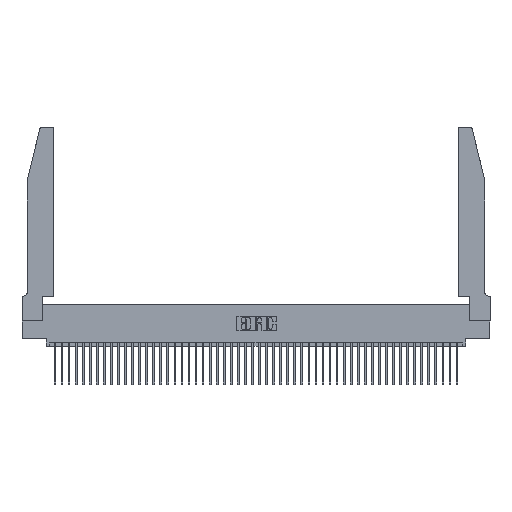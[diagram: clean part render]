
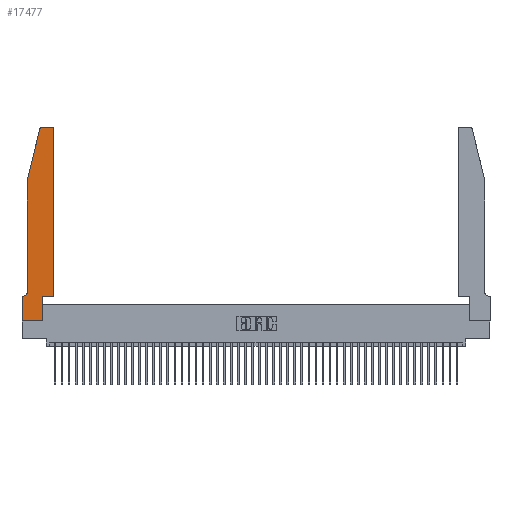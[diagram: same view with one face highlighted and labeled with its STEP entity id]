
A CAD part, top view. The second image highlights one B-rep face of the part: STEP entity #17477.
In plain terms, the highlighted planar face has unit normal (0, 0, 1).
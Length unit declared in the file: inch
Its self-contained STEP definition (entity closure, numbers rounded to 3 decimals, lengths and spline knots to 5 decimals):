
#53 = VERTEX_POINT ( 'NONE', #31183 ) ;
#1269 = CIRCLE ( 'NONE', #37460, 0.03 ) ;
#1338 = CARTESIAN_POINT ( 'NONE',  ( 0.4505, 0.35, 0.37 ) ) ;
#1360 = DIRECTION ( 'NONE',  ( 0., 0., 1. ) ) ;
#1592 = VECTOR ( 'NONE', #30596, 39.37008 ) ;
#1834 = VERTEX_POINT ( 'NONE', #38610 ) ;
#2089 = ORIENTED_EDGE ( 'NONE', *, *, #30046, .T. ) ;
#3142 = VERTEX_POINT ( 'NONE', #16847 ) ;
#4029 = EDGE_CURVE ( 'NONE', #45872, #11763, #17822, .T. ) ;
#4580 = ORIENTED_EDGE ( 'NONE', *, *, #7822, .T. ) ;
#5085 = PLANE ( 'NONE',  #37215 ) ;
#5420 = EDGE_CURVE ( 'NONE', #19648, #16205, #38707, .T. ) ;
#5637 = VERTEX_POINT ( 'NONE', #30866 ) ;
#6032 = ORIENTED_EDGE ( 'NONE', *, *, #9380, .T. ) ;
#7026 = ORIENTED_EDGE ( 'NONE', *, *, #36042, .T. ) ;
#7822 = EDGE_CURVE ( 'NONE', #3142, #5637, #47270, .T. ) ;
#8470 = VECTOR ( 'NONE', #11796, 39.37008 ) ;
#8749 = CARTESIAN_POINT ( 'NONE',  ( 0.2865, 0.35, 0.37 ) ) ;
#9177 = CARTESIAN_POINT ( 'NONE',  ( 0.0055, 0.42, 0.37 ) ) ;
#9285 = EDGE_CURVE ( 'NONE', #36598, #53, #1269, .T. ) ;
#9380 = EDGE_CURVE ( 'NONE', #31233, #19648, #23908, .T. ) ;
#9903 = ORIENTED_EDGE ( 'NONE', *, *, #30215, .T. ) ;
#10704 = VERTEX_POINT ( 'NONE', #27203 ) ;
#11409 = LINE ( 'NONE', #30130, #20197 ) ;
#11763 = VERTEX_POINT ( 'NONE', #32856 ) ;
#11796 = DIRECTION ( 'NONE',  ( -1., 0., 0. ) ) ;
#12970 = EDGE_CURVE ( 'NONE', #10704, #45872, #26565, .T. ) ;
#13613 = VERTEX_POINT ( 'NONE', #40194 ) ;
#15074 = VECTOR ( 'NONE', #30107, 39.37008 ) ;
#15516 = CARTESIAN_POINT ( 'NONE',  ( 0.4505, 0.35, 0.37 ) ) ;
#15694 = DIRECTION ( 'NONE',  ( 1., 0., 0. ) ) ;
#16205 = VERTEX_POINT ( 'NONE', #39256 ) ;
#16847 = CARTESIAN_POINT ( 'NONE',  ( 0.2865, 0., 0.37 ) ) ;
#17477 = ADVANCED_FACE ( 'NONE', ( #25300 ), #5085, .T. ) ;
#17822 = CIRCLE ( 'NONE', #23150, 0.03 ) ;
#17954 = ORIENTED_EDGE ( 'NONE', *, *, #9285, .T. ) ;
#19648 = VERTEX_POINT ( 'NONE', #41262 ) ;
#20080 = DIRECTION ( 'NONE',  ( 1., 0., 0. ) ) ;
#20197 = VECTOR ( 'NONE', #45493, 39.37008 ) ;
#20607 = VECTOR ( 'NONE', #45536, 39.37008 ) ;
#20691 = VECTOR ( 'NONE', #45403, 39.37008 ) ;
#21828 = LINE ( 'NONE', #23031, #20691 ) ;
#23022 = EDGE_CURVE ( 'NONE', #16205, #13613, #11409, .T. ) ;
#23031 = CARTESIAN_POINT ( 'NONE',  ( 0.0755, 2., 0.37 ) ) ;
#23150 = AXIS2_PLACEMENT_3D ( 'NONE', #26439, #41498, #15694 ) ;
#23663 = DIRECTION ( 'NONE',  ( 0., 0., -1. ) ) ;
#23764 = CARTESIAN_POINT ( 'NONE',  ( 0., 0.35, 0.37 ) ) ;
#23908 = CIRCLE ( 'NONE', #37174, 0.07 ) ;
#24202 = EDGE_CURVE ( 'NONE', #53, #1834, #21828, .T. ) ;
#24320 = ORIENTED_EDGE ( 'NONE', *, *, #23022, .T. ) ;
#24430 = CARTESIAN_POINT ( 'NONE',  ( 0.284, 2.72, 0.37 ) ) ;
#25300 = FACE_OUTER_BOUND ( 'NONE', #26370, .T. ) ;
#26370 = EDGE_LOOP ( 'NONE', ( #7026, #17954, #39150, #9903, #6032, #30390, #24320, #47570, #4580, #2089, #48081, #40801 ) ) ;
#26439 = CARTESIAN_POINT ( 'NONE',  ( 0.4205, 2.72, 0.37 ) ) ;
#26565 = LINE ( 'NONE', #1338, #48169 ) ;
#26760 = CARTESIAN_POINT ( 'NONE',  ( 0.4505, 2.72, 0.37 ) ) ;
#27203 = CARTESIAN_POINT ( 'NONE',  ( 0.4505, 0.35, 0.37 ) ) ;
#28224 = DIRECTION ( 'NONE',  ( 0., 0., 1. ) ) ;
#28835 = EDGE_CURVE ( 'NONE', #13613, #3142, #38444, .T. ) ;
#30027 = CARTESIAN_POINT ( 'NONE',  ( 0.2605, 2.75, 0.37 ) ) ;
#30046 = EDGE_CURVE ( 'NONE', #5637, #10704, #33677, .T. ) ;
#30107 = DIRECTION ( 'NONE',  ( 1., 0., 0. ) ) ;
#30130 = CARTESIAN_POINT ( 'NONE',  ( 0., 0., 0.37 ) ) ;
#30215 = EDGE_CURVE ( 'NONE', #1834, #31233, #47066, .T. ) ;
#30390 = ORIENTED_EDGE ( 'NONE', *, *, #5420, .T. ) ;
#30596 = DIRECTION ( 'NONE',  ( 0., -1., 0. ) ) ;
#30866 = CARTESIAN_POINT ( 'NONE',  ( 0.2865, 0.35, 0.37 ) ) ;
#31110 = DIRECTION ( 'NONE',  ( 0., 1., 0. ) ) ;
#31183 = CARTESIAN_POINT ( 'NONE',  ( 0.25487, 2.72718, 0.37 ) ) ;
#31233 = VERTEX_POINT ( 'NONE', #35747 ) ;
#32856 = CARTESIAN_POINT ( 'NONE',  ( 0.4205, 2.75, 0.37 ) ) ;
#33460 = DIRECTION ( 'NONE',  ( 1., 0., 0. ) ) ;
#33469 = CARTESIAN_POINT ( 'NONE',  ( 0.0755, 0.35, 0.37 ) ) ;
#33677 = LINE ( 'NONE', #15516, #40097 ) ;
#35747 = CARTESIAN_POINT ( 'NONE',  ( 0.0755, 0.42, 0.37 ) ) ;
#36042 = EDGE_CURVE ( 'NONE', #11763, #36598, #48152, .T. ) ;
#36598 = VERTEX_POINT ( 'NONE', #44968 ) ;
#37174 = AXIS2_PLACEMENT_3D ( 'NONE', #9177, #23663, #38232 ) ;
#37215 = AXIS2_PLACEMENT_3D ( 'NONE', #23764, #1360, #20080 ) ;
#37315 = CARTESIAN_POINT ( 'NONE',  ( 0., 0., 0.37 ) ) ;
#37460 = AXIS2_PLACEMENT_3D ( 'NONE', #24430, #28224, #43240 ) ;
#38232 = DIRECTION ( 'NONE',  ( -1., 0., 0. ) ) ;
#38444 = LINE ( 'NONE', #37315, #15074 ) ;
#38610 = CARTESIAN_POINT ( 'NONE',  ( 0.0755, 2., 0.37 ) ) ;
#38707 = LINE ( 'NONE', #33469, #20607 ) ;
#39150 = ORIENTED_EDGE ( 'NONE', *, *, #24202, .T. ) ;
#39256 = CARTESIAN_POINT ( 'NONE',  ( 0., 0.35, 0.37 ) ) ;
#40097 = VECTOR ( 'NONE', #33460, 39.37008 ) ;
#40194 = CARTESIAN_POINT ( 'NONE',  ( 0., 0., 0.37 ) ) ;
#40801 = ORIENTED_EDGE ( 'NONE', *, *, #4029, .T. ) ;
#41262 = CARTESIAN_POINT ( 'NONE',  ( 0.0055, 0.35, 0.37 ) ) ;
#41498 = DIRECTION ( 'NONE',  ( 0., 0., 1. ) ) ;
#43240 = DIRECTION ( 'NONE',  ( 1., 0., 0. ) ) ;
#44968 = CARTESIAN_POINT ( 'NONE',  ( 0.284, 2.75, 0.37 ) ) ;
#45403 = DIRECTION ( 'NONE',  ( -0.239, -0.971, 0. ) ) ;
#45493 = DIRECTION ( 'NONE',  ( 0., -1., 0. ) ) ;
#45536 = DIRECTION ( 'NONE',  ( -1., 0., 0. ) ) ;
#45556 = VECTOR ( 'NONE', #47699, 39.37008 ) ;
#45872 = VERTEX_POINT ( 'NONE', #26760 ) ;
#45934 = CARTESIAN_POINT ( 'NONE',  ( 0.0755, 2., 0.37 ) ) ;
#47066 = LINE ( 'NONE', #45934, #1592 ) ;
#47270 = LINE ( 'NONE', #8749, #45556 ) ;
#47570 = ORIENTED_EDGE ( 'NONE', *, *, #28835, .T. ) ;
#47699 = DIRECTION ( 'NONE',  ( 0., 1., 0. ) ) ;
#48081 = ORIENTED_EDGE ( 'NONE', *, *, #12970, .T. ) ;
#48152 = LINE ( 'NONE', #30027, #8470 ) ;
#48169 = VECTOR ( 'NONE', #31110, 39.37008 ) ;
